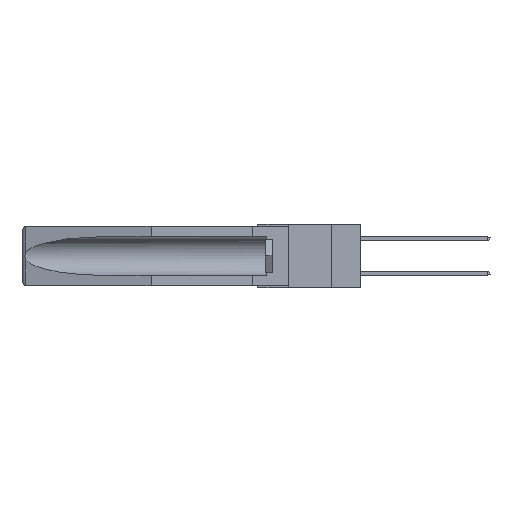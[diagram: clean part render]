
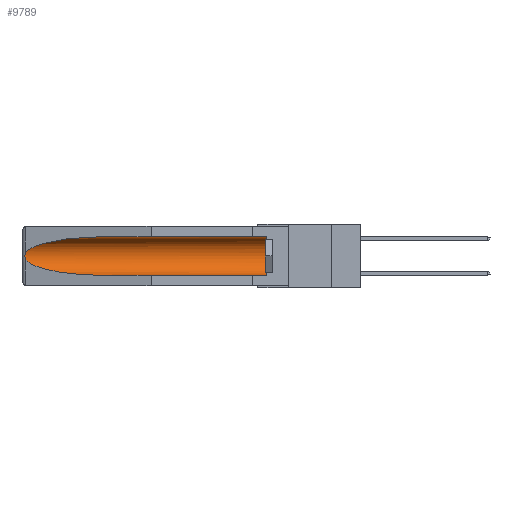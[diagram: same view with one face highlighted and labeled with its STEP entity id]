
A CAD part, left-side view. The second image highlights one B-rep face of the part: STEP entity #9789.
In plain terms, the highlighted cylindrical face has radius 2.857 mm (diameter 5.715 mm), a partial arc.
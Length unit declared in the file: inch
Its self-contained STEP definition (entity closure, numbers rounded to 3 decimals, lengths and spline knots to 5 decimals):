
#56 = CARTESIAN_POINT ( 'NONE',  ( 0.155, 0.126, -0.284 ) ) ;
#1147 = ORIENTED_EDGE ( 'NONE', *, *, #13485, .T. ) ;
#1805 = CIRCLE ( 'NONE', #13282, 0.1125 ) ;
#2961 = CARTESIAN_POINT ( 'NONE',  ( 0.26597, 1.52961, -0.15275 ) ) ;
#3498 = B_SPLINE_CURVE_WITH_KNOTS ( 'NONE', 3,
 ( #25571, #2961, #23471, #7216, #5062, #21554, #17480, #23389, #9005, #23210 ),
 .UNSPECIFIED., .F., .F.,
 ( 4, 2, 2, 2, 4 ),
 ( 0., 0.00029, 0.00058, 0.00087, 0.00117 ),
 .UNSPECIFIED. ) ;
#3696 = CARTESIAN_POINT ( 'NONE',  ( 0.21114, 1.30732, -0.284 ) ) ;
#3822 =( BOUNDED_CURVE ( )  B_SPLINE_CURVE ( 3, ( #20263, #12140, #3934, #18265 ),
 .UNSPECIFIED., .F., .F. ) 
 B_SPLINE_CURVE_WITH_KNOTS ( ( 4, 4 ),
 ( 4.71239, 6.08839 ),
 .UNSPECIFIED. ) 
 CURVE ( )  GEOMETRIC_REPRESENTATION_ITEM ( )  RATIONAL_B_SPLINE_CURVE ( ( 1., 0.848, 0.848, 1. ) ) 
 REPRESENTATION_ITEM ( '' )  );
#3934 = CARTESIAN_POINT ( 'NONE',  ( 0.25451, 1.48313, -0.09465 ) ) ;
#4429 = ORIENTED_EDGE ( 'NONE', *, *, #4778, .T. ) ;
#4778 = EDGE_CURVE ( 'NONE', #6778, #7016, #1805, .T. ) ;
#4994 = VECTOR ( 'NONE', #21803, 39.37008 ) ;
#5005 = VERTEX_POINT ( 'NONE', #9998 ) ;
#5062 = CARTESIAN_POINT ( 'NONE',  ( 0.2675, 1.53308, -0.16763 ) ) ;
#5699 = DIRECTION ( 'NONE',  ( 0., 0., 1. ) ) ;
#5709 = CARTESIAN_POINT ( 'NONE',  ( 0.155, 1.07973, -0.284 ) ) ;
#6401 = CARTESIAN_POINT ( 'NONE',  ( 0.155, -0.30754, -0.284 ) ) ;
#6778 = VERTEX_POINT ( 'NONE', #56 ) ;
#7016 = VERTEX_POINT ( 'NONE', #12827 ) ;
#7216 = CARTESIAN_POINT ( 'NONE',  ( 0.2673, 1.5327, -0.16383 ) ) ;
#7884 = CARTESIAN_POINT ( 'NONE',  ( 0.26537, 1.52718, -0.19328 ) ) ;
#7923 = EDGE_CURVE ( 'NONE', #26224, #16175, #18124, .T. ) ;
#8289 = CARTESIAN_POINT ( 'NONE',  ( 0.155, 0.126, -0.1715 ) ) ;
#8677 = LINE ( 'NONE', #6401, #25999 ) ;
#8939 = CARTESIAN_POINT ( 'NONE',  ( 0.155, 1.07973, -0.059 ) ) ;
#9005 = CARTESIAN_POINT ( 'NONE',  ( 0.26597, 1.5296, -0.19026 ) ) ;
#9789 = ADVANCED_FACE ( 'NONE', ( #25501 ), #22310, .F. ) ;
#9998 = CARTESIAN_POINT ( 'NONE',  ( 0.26537, 1.52718, -0.14972 ) ) ;
#10035 = EDGE_LOOP ( 'NONE', ( #1147, #13027, #10111, #15073, #4429, #21669 ) ) ;
#10111 = ORIENTED_EDGE ( 'NONE', *, *, #7923, .T. ) ;
#10467 = EDGE_CURVE ( 'NONE', #5005, #26224, #3498, .T. ) ;
#10477 = LINE ( 'NONE', #25743, #4994 ) ;
#11161 = DIRECTION ( 'NONE',  ( 0., 0., 1. ) ) ;
#12140 = CARTESIAN_POINT ( 'NONE',  ( 0.21114, 1.30732, -0.059 ) ) ;
#12355 = DIRECTION ( 'NONE',  ( 0., 1., 0. ) ) ;
#12827 = CARTESIAN_POINT ( 'NONE',  ( 0.155, 0.126, -0.059 ) ) ;
#12886 = EDGE_CURVE ( 'NONE', #7016, #14094, #10477, .T. ) ;
#13027 = ORIENTED_EDGE ( 'NONE', *, *, #10467, .T. ) ;
#13282 = AXIS2_PLACEMENT_3D ( 'NONE', #8289, #23831, #5699 ) ;
#13485 = EDGE_CURVE ( 'NONE', #14094, #5005, #3822, .T. ) ;
#14040 = CARTESIAN_POINT ( 'NONE',  ( 0.26537, 1.52718, -0.19328 ) ) ;
#14094 = VERTEX_POINT ( 'NONE', #8939 ) ;
#15073 = ORIENTED_EDGE ( 'NONE', *, *, #26399, .F. ) ;
#15212 = CARTESIAN_POINT ( 'NONE',  ( 0.155, 1.07973, -0.284 ) ) ;
#16175 = VERTEX_POINT ( 'NONE', #15212 ) ;
#17480 = CARTESIAN_POINT ( 'NONE',  ( 0.2673, 1.53269, -0.17917 ) ) ;
#18124 =( BOUNDED_CURVE ( )  B_SPLINE_CURVE ( 3, ( #14040, #26135, #3696, #5709 ),
 .UNSPECIFIED., .F., .F. ) 
 B_SPLINE_CURVE_WITH_KNOTS ( ( 4, 4 ),
 ( 0.1948, 1.5708 ),
 .UNSPECIFIED. ) 
 CURVE ( )  GEOMETRIC_REPRESENTATION_ITEM ( )  RATIONAL_B_SPLINE_CURVE ( ( 1., 0.848, 0.848, 1. ) ) 
 REPRESENTATION_ITEM ( '' )  );
#18265 = CARTESIAN_POINT ( 'NONE',  ( 0.26537, 1.52718, -0.14972 ) ) ;
#19702 = AXIS2_PLACEMENT_3D ( 'NONE', #22912, #23280, #11161 ) ;
#20263 = CARTESIAN_POINT ( 'NONE',  ( 0.155, 1.07973, -0.059 ) ) ;
#21554 = CARTESIAN_POINT ( 'NONE',  ( 0.2675, 1.53308, -0.17534 ) ) ;
#21669 = ORIENTED_EDGE ( 'NONE', *, *, #12886, .T. ) ;
#21803 = DIRECTION ( 'NONE',  ( 0., 1., 0. ) ) ;
#22310 = CYLINDRICAL_SURFACE ( 'NONE', #19702, 0.1125 ) ;
#22912 = CARTESIAN_POINT ( 'NONE',  ( 0.155, -0.30754, -0.1715 ) ) ;
#23210 = CARTESIAN_POINT ( 'NONE',  ( 0.26537, 1.52718, -0.19328 ) ) ;
#23280 = DIRECTION ( 'NONE',  ( 0., 1., 0. ) ) ;
#23389 = CARTESIAN_POINT ( 'NONE',  ( 0.26655, 1.53094, -0.18657 ) ) ;
#23471 = CARTESIAN_POINT ( 'NONE',  ( 0.26654, 1.53092, -0.15636 ) ) ;
#23831 = DIRECTION ( 'NONE',  ( 0., -1., 0. ) ) ;
#25501 = FACE_OUTER_BOUND ( 'NONE', #10035, .T. ) ;
#25571 = CARTESIAN_POINT ( 'NONE',  ( 0.26537, 1.52718, -0.14972 ) ) ;
#25743 = CARTESIAN_POINT ( 'NONE',  ( 0.155, -0.30754, -0.059 ) ) ;
#25999 = VECTOR ( 'NONE', #12355, 39.37008 ) ;
#26135 = CARTESIAN_POINT ( 'NONE',  ( 0.25451, 1.48313, -0.24835 ) ) ;
#26224 = VERTEX_POINT ( 'NONE', #7884 ) ;
#26399 = EDGE_CURVE ( 'NONE', #6778, #16175, #8677, .T. ) ;
